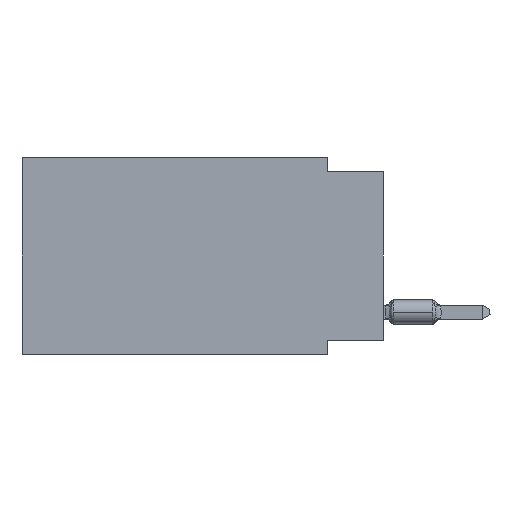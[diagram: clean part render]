
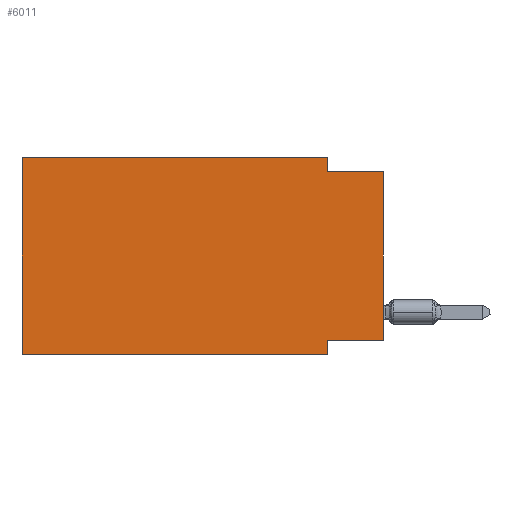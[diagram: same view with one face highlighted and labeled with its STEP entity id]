
A CAD part, left-side view. The second image highlights one B-rep face of the part: STEP entity #6011.
In plain terms, the highlighted planar face has unit normal (-1, 0, 0).
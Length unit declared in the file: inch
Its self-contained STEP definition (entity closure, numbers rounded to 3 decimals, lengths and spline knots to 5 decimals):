
#22 = VERTEX_POINT ( 'NONE', #212 ) ;
#84 = DIRECTION ( 'NONE',  ( 0., -1., 0. ) ) ;
#212 = CARTESIAN_POINT ( 'NONE',  ( 0., 0.645, 0. ) ) ;
#1090 = CARTESIAN_POINT ( 'NONE',  ( 0., 0.645, 0. ) ) ;
#1594 = ORIENTED_EDGE ( 'NONE', *, *, #20407, .T. ) ;
#1603 = ORIENTED_EDGE ( 'NONE', *, *, #2755, .F. ) ;
#2384 = CARTESIAN_POINT ( 'NONE',  ( 0., 0., -0.325 ) ) ;
#2755 = EDGE_CURVE ( 'NONE', #16017, #3608, #16012, .T. ) ;
#2949 = EDGE_CURVE ( 'NONE', #22, #16017, #23497, .T. ) ;
#3608 = VERTEX_POINT ( 'NONE', #3959 ) ;
#3944 = LINE ( 'NONE', #11983, #20882 ) ;
#3959 = CARTESIAN_POINT ( 'NONE',  ( 0., 0.1, -0.025 ) ) ;
#4239 = CARTESIAN_POINT ( 'NONE',  ( 0., 0.645, -0.35 ) ) ;
#4909 = VERTEX_POINT ( 'NONE', #17848 ) ;
#5119 = LINE ( 'NONE', #21627, #14192 ) ;
#5428 = EDGE_LOOP ( 'NONE', ( #24219, #13579, #1603, #8088, #5626, #1594, #6310, #21552 ) ) ;
#5626 = ORIENTED_EDGE ( 'NONE', *, *, #19895, .F. ) ;
#6011 = ADVANCED_FACE ( 'NONE', ( #8871 ), #23994, .F. ) ;
#6310 = ORIENTED_EDGE ( 'NONE', *, *, #7562, .F. ) ;
#6535 = LINE ( 'NONE', #20844, #19220 ) ;
#6610 = EDGE_CURVE ( 'NONE', #11424, #4909, #26527, .T. ) ;
#6818 = LINE ( 'NONE', #17174, #21269 ) ;
#7305 = DIRECTION ( 'NONE',  ( 0., -1., 0. ) ) ;
#7562 = EDGE_CURVE ( 'NONE', #4909, #26699, #6535, .T. ) ;
#7846 = CARTESIAN_POINT ( 'NONE',  ( 0., 0., -0.325 ) ) ;
#8088 = ORIENTED_EDGE ( 'NONE', *, *, #2949, .F. ) ;
#8871 = FACE_OUTER_BOUND ( 'NONE', #5428, .T. ) ;
#9141 = DIRECTION ( 'NONE',  ( 1., 0., 0. ) ) ;
#11140 = EDGE_CURVE ( 'NONE', #3608, #22650, #5119, .T. ) ;
#11424 = VERTEX_POINT ( 'NONE', #2384 ) ;
#11490 = VECTOR ( 'NONE', #24326, 39.37008 ) ;
#11983 = CARTESIAN_POINT ( 'NONE',  ( 0., 0.645, 0. ) ) ;
#12114 = DIRECTION ( 'NONE',  ( 0., 0., 1. ) ) ;
#13058 = VECTOR ( 'NONE', #14607, 39.37008 ) ;
#13151 = CARTESIAN_POINT ( 'NONE',  ( 0., 0.645, 0. ) ) ;
#13579 = ORIENTED_EDGE ( 'NONE', *, *, #11140, .F. ) ;
#13974 = CARTESIAN_POINT ( 'NONE',  ( 0., 0.1, 0. ) ) ;
#14112 = CARTESIAN_POINT ( 'NONE',  ( 0., 0.1, -0.35 ) ) ;
#14192 = VECTOR ( 'NONE', #7305, 39.37008 ) ;
#14607 = DIRECTION ( 'NONE',  ( 0., -1., 0. ) ) ;
#15012 = LINE ( 'NONE', #4239, #13058 ) ;
#15121 = DIRECTION ( 'NONE',  ( 0., 0., 1. ) ) ;
#16012 = LINE ( 'NONE', #13974, #11490 ) ;
#16017 = VERTEX_POINT ( 'NONE', #23795 ) ;
#17174 = CARTESIAN_POINT ( 'NONE',  ( 0., 0., 0. ) ) ;
#17361 = EDGE_CURVE ( 'NONE', #11424, #22650, #6818, .T. ) ;
#17436 = VECTOR ( 'NONE', #24483, 39.37008 ) ;
#17468 = DIRECTION ( 'NONE',  ( 0., 0., -1. ) ) ;
#17848 = CARTESIAN_POINT ( 'NONE',  ( 0., 0.1, -0.325 ) ) ;
#18815 = DIRECTION ( 'NONE',  ( 0., 0., -1. ) ) ;
#19220 = VECTOR ( 'NONE', #18815, 39.37008 ) ;
#19849 = CARTESIAN_POINT ( 'NONE',  ( 0., 0., -0.025 ) ) ;
#19895 = EDGE_CURVE ( 'NONE', #23513, #22, #3944, .T. ) ;
#20011 = CARTESIAN_POINT ( 'NONE',  ( 0., 0.645, -0.35 ) ) ;
#20190 = AXIS2_PLACEMENT_3D ( 'NONE', #1090, #9141, #17468 ) ;
#20407 = EDGE_CURVE ( 'NONE', #23513, #26699, #15012, .T. ) ;
#20844 = CARTESIAN_POINT ( 'NONE',  ( 0., 0.1, -0.35 ) ) ;
#20882 = VECTOR ( 'NONE', #12114, 39.37008 ) ;
#21119 = VECTOR ( 'NONE', #84, 39.37008 ) ;
#21269 = VECTOR ( 'NONE', #15121, 39.37008 ) ;
#21552 = ORIENTED_EDGE ( 'NONE', *, *, #6610, .F. ) ;
#21627 = CARTESIAN_POINT ( 'NONE',  ( 0., 0., -0.025 ) ) ;
#22650 = VERTEX_POINT ( 'NONE', #19849 ) ;
#23497 = LINE ( 'NONE', #13151, #21119 ) ;
#23513 = VERTEX_POINT ( 'NONE', #20011 ) ;
#23795 = CARTESIAN_POINT ( 'NONE',  ( 0., 0.1, 0. ) ) ;
#23994 = PLANE ( 'NONE',  #20190 ) ;
#24219 = ORIENTED_EDGE ( 'NONE', *, *, #17361, .T. ) ;
#24326 = DIRECTION ( 'NONE',  ( 0., 0., -1. ) ) ;
#24483 = DIRECTION ( 'NONE',  ( 0., 1., 0. ) ) ;
#26527 = LINE ( 'NONE', #7846, #17436 ) ;
#26699 = VERTEX_POINT ( 'NONE', #14112 ) ;
